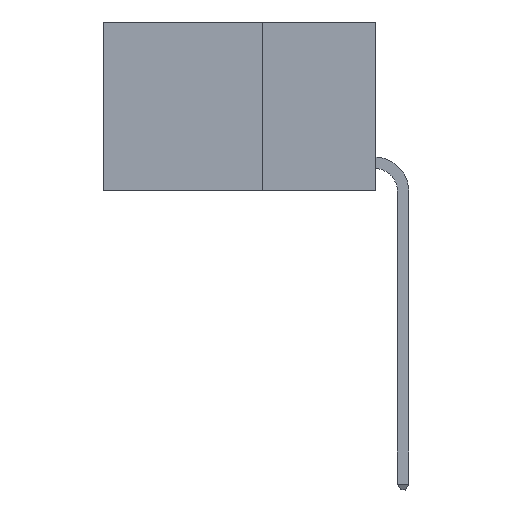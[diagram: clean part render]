
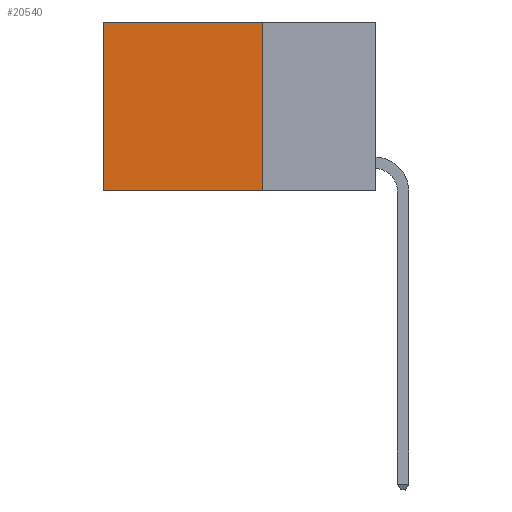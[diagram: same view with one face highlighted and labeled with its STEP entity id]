
A CAD part, left-side view. The second image highlights one B-rep face of the part: STEP entity #20540.
In plain terms, the highlighted planar face has unit normal (-1, 0, 0).
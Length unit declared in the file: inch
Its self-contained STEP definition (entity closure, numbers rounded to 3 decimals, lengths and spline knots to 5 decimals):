
#685 = LINE ( 'NONE', #3169, #10359 ) ;
#851 = FACE_OUTER_BOUND ( 'NONE', #9768, .T. ) ;
#1639 = AXIS2_PLACEMENT_3D ( 'NONE', #1771, #15237, #3708 ) ;
#1771 = CARTESIAN_POINT ( 'NONE',  ( 0.2625, 0.25, 0. ) ) ;
#2044 = VECTOR ( 'NONE', #11465, 39.37008 ) ;
#2323 = CARTESIAN_POINT ( 'NONE',  ( 0.2625, 0.6, -0.37 ) ) ;
#2666 = LINE ( 'NONE', #17118, #2044 ) ;
#3169 = CARTESIAN_POINT ( 'NONE',  ( 0.2625, 0.25, 0. ) ) ;
#3178 = VERTEX_POINT ( 'NONE', #11960 ) ;
#3708 = DIRECTION ( 'NONE',  ( 0., 0., -1. ) ) ;
#4088 = DIRECTION ( 'NONE',  ( 0., 0., -1. ) ) ;
#4141 = CARTESIAN_POINT ( 'NONE',  ( 0.2625, 0.25, -0.37 ) ) ;
#4321 = EDGE_CURVE ( 'NONE', #8721, #12848, #2666, .T. ) ;
#4887 = VERTEX_POINT ( 'NONE', #4141 ) ;
#5094 = DIRECTION ( 'NONE',  ( 0., 1., 0. ) ) ;
#5315 = VECTOR ( 'NONE', #20468, 39.37008 ) ;
#8721 = VERTEX_POINT ( 'NONE', #17055 ) ;
#8873 = VECTOR ( 'NONE', #4088, 39.37008 ) ;
#9104 = CARTESIAN_POINT ( 'NONE',  ( 0.2625, 0.25, -0.37 ) ) ;
#9482 = LINE ( 'NONE', #21193, #8873 ) ;
#9768 = EDGE_LOOP ( 'NONE', ( #13463, #13510, #13617, #13645 ) ) ;
#10359 = VECTOR ( 'NONE', #5094, 39.37008 ) ;
#11080 = LINE ( 'NONE', #9104, #5315 ) ;
#11465 = DIRECTION ( 'NONE',  ( 0., 0., -1. ) ) ;
#11960 = CARTESIAN_POINT ( 'NONE',  ( 0.2625, 0.25, 0. ) ) ;
#12848 = VERTEX_POINT ( 'NONE', #2323 ) ;
#13463 = ORIENTED_EDGE ( 'NONE', *, *, #4321, .T. ) ;
#13510 = ORIENTED_EDGE ( 'NONE', *, *, #15624, .F. ) ;
#13617 = ORIENTED_EDGE ( 'NONE', *, *, #17140, .F. ) ;
#13645 = ORIENTED_EDGE ( 'NONE', *, *, #24695, .T. ) ;
#15237 = DIRECTION ( 'NONE',  ( 1., 0., 0. ) ) ;
#15624 = EDGE_CURVE ( 'NONE', #4887, #12848, #11080, .T. ) ;
#17055 = CARTESIAN_POINT ( 'NONE',  ( 0.2625, 0.6, 0. ) ) ;
#17118 = CARTESIAN_POINT ( 'NONE',  ( 0.2625, 0.6, 0. ) ) ;
#17140 = EDGE_CURVE ( 'NONE', #3178, #4887, #9482, .T. ) ;
#20468 = DIRECTION ( 'NONE',  ( 0., 1., 0. ) ) ;
#20540 = ADVANCED_FACE ( 'NONE', ( #851 ), #20811, .F. ) ;
#20811 = PLANE ( 'NONE',  #1639 ) ;
#21193 = CARTESIAN_POINT ( 'NONE',  ( 0.2625, 0.25, 0. ) ) ;
#24695 = EDGE_CURVE ( 'NONE', #3178, #8721, #685, .T. ) ;
